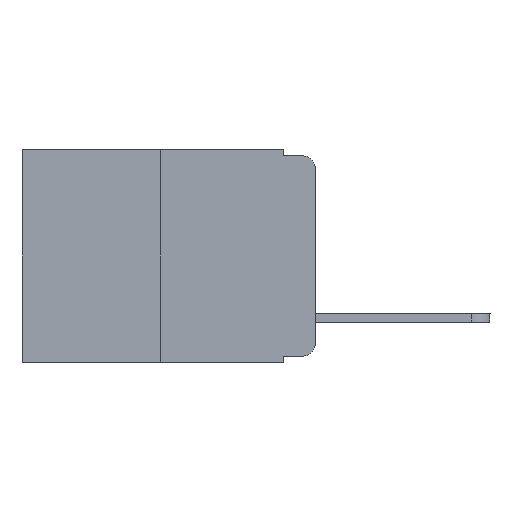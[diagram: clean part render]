
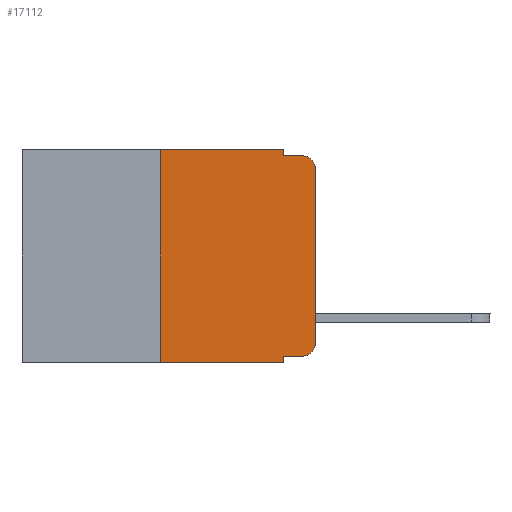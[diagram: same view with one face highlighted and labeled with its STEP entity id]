
A CAD part, left-side view. The second image highlights one B-rep face of the part: STEP entity #17112.
In plain terms, the highlighted planar face has unit normal (-1, 0, 0).
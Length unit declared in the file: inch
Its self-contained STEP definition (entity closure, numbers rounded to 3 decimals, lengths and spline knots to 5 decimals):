
#529 = CARTESIAN_POINT ( 'NONE',  ( 0., 0.051, -0.01 ) ) ;
#1294 = ORIENTED_EDGE ( 'NONE', *, *, #14803, .T. ) ;
#1505 = CIRCLE ( 'NONE', #15789, 0.02 ) ;
#2077 = CIRCLE ( 'NONE', #4795, 0.02 ) ;
#2731 = DIRECTION ( 'NONE',  ( 0., -1., 0. ) ) ;
#3553 = ORIENTED_EDGE ( 'NONE', *, *, #17590, .T. ) ;
#3739 = EDGE_LOOP ( 'NONE', ( #15089, #13191, #12401, #16859, #12333, #10802, #3553, #10987, #18357, #1294 ) ) ;
#4099 = DIRECTION ( 'NONE',  ( 0., 0., -1. ) ) ;
#4581 = VERTEX_POINT ( 'NONE', #529 ) ;
#4795 = AXIS2_PLACEMENT_3D ( 'NONE', #14480, #7601, #9352 ) ;
#4828 = DIRECTION ( 'NONE',  ( 0., 0., -1. ) ) ;
#4833 = CARTESIAN_POINT ( 'NONE',  ( 0., 0., -0.03 ) ) ;
#4875 = DIRECTION ( 'NONE',  ( 0., 0., -1. ) ) ;
#5605 = VECTOR ( 'NONE', #14605, 39.37008 ) ;
#5827 = CARTESIAN_POINT ( 'NONE',  ( 0., 0.25, 0. ) ) ;
#6003 = EDGE_CURVE ( 'NONE', #11993, #21894, #17107, .T. ) ;
#6407 = VERTEX_POINT ( 'NONE', #6464 ) ;
#6464 = CARTESIAN_POINT ( 'NONE',  ( 0., 0.02, -0.333 ) ) ;
#7314 = CARTESIAN_POINT ( 'NONE',  ( 0., 0.02, -0.313 ) ) ;
#7601 = DIRECTION ( 'NONE',  ( -1., 0., 0. ) ) ;
#7742 = VECTOR ( 'NONE', #12915, 39.37008 ) ;
#8338 = PLANE ( 'NONE',  #21215 ) ;
#9352 = DIRECTION ( 'NONE',  ( 0., 0., -1. ) ) ;
#9434 = DIRECTION ( 'NONE',  ( 0., -1., 0. ) ) ;
#9860 = EDGE_CURVE ( 'NONE', #4581, #17073, #19650, .T. ) ;
#9928 = VECTOR ( 'NONE', #18973, 39.37008 ) ;
#10130 = VERTEX_POINT ( 'NONE', #19594 ) ;
#10802 = ORIENTED_EDGE ( 'NONE', *, *, #18186, .F. ) ;
#10987 = ORIENTED_EDGE ( 'NONE', *, *, #6003, .F. ) ;
#11107 = CARTESIAN_POINT ( 'NONE',  ( 0., 0.473, -0.343 ) ) ;
#11209 = CARTESIAN_POINT ( 'NONE',  ( 0., 0.051, -0.333 ) ) ;
#11373 = VERTEX_POINT ( 'NONE', #4833 ) ;
#11555 = LINE ( 'NONE', #15477, #9928 ) ;
#11988 = VECTOR ( 'NONE', #4828, 39.37008 ) ;
#11993 = VERTEX_POINT ( 'NONE', #11209 ) ;
#12045 = CARTESIAN_POINT ( 'NONE',  ( 0., 0., -0.313 ) ) ;
#12333 = ORIENTED_EDGE ( 'NONE', *, *, #15250, .F. ) ;
#12401 = ORIENTED_EDGE ( 'NONE', *, *, #9860, .F. ) ;
#12915 = DIRECTION ( 'NONE',  ( 0., 0., 1. ) ) ;
#12977 = FACE_OUTER_BOUND ( 'NONE', #3739, .T. ) ;
#13163 = LINE ( 'NONE', #13746, #13716 ) ;
#13191 = ORIENTED_EDGE ( 'NONE', *, *, #17573, .T. ) ;
#13472 = CARTESIAN_POINT ( 'NONE',  ( 0., 0.473, 0. ) ) ;
#13675 = DIRECTION ( 'NONE',  ( 0., 0., -1. ) ) ;
#13716 = VECTOR ( 'NONE', #13675, 39.37008 ) ;
#13746 = CARTESIAN_POINT ( 'NONE',  ( 0., 0.051, 0. ) ) ;
#14480 = CARTESIAN_POINT ( 'NONE',  ( 0., 0.02, -0.03 ) ) ;
#14586 = CARTESIAN_POINT ( 'NONE',  ( 0., 0.051, -0.333 ) ) ;
#14605 = DIRECTION ( 'NONE',  ( 0., 0., 1. ) ) ;
#14635 = VERTEX_POINT ( 'NONE', #12045 ) ;
#14786 = CARTESIAN_POINT ( 'NONE',  ( 0., 0.051, 0. ) ) ;
#14803 = EDGE_CURVE ( 'NONE', #6407, #14635, #1505, .T. ) ;
#14926 = EDGE_CURVE ( 'NONE', #14635, #11373, #19141, .T. ) ;
#15005 = CARTESIAN_POINT ( 'NONE',  ( 0., 0.25, -0.343 ) ) ;
#15089 = ORIENTED_EDGE ( 'NONE', *, *, #14926, .T. ) ;
#15250 = EDGE_CURVE ( 'NONE', #10130, #17702, #11555, .T. ) ;
#15280 = EDGE_CURVE ( 'NONE', #17702, #4581, #13163, .T. ) ;
#15477 = CARTESIAN_POINT ( 'NONE',  ( 0., 0.473, 0. ) ) ;
#15673 = VERTEX_POINT ( 'NONE', #15005 ) ;
#15716 = CARTESIAN_POINT ( 'NONE',  ( 0., 0.051, -0.01 ) ) ;
#15789 = AXIS2_PLACEMENT_3D ( 'NONE', #7314, #16079, #4099 ) ;
#16079 = DIRECTION ( 'NONE',  ( -1., 0., 0. ) ) ;
#16113 = VECTOR ( 'NONE', #21182, 39.37008 ) ;
#16307 = CARTESIAN_POINT ( 'NONE',  ( 0., 0., 0. ) ) ;
#16730 = CARTESIAN_POINT ( 'NONE',  ( 0., 0.051, 0. ) ) ;
#16859 = ORIENTED_EDGE ( 'NONE', *, *, #15280, .F. ) ;
#17055 = EDGE_CURVE ( 'NONE', #11993, #6407, #18686, .T. ) ;
#17073 = VERTEX_POINT ( 'NONE', #20537 ) ;
#17107 = LINE ( 'NONE', #16730, #11988 ) ;
#17112 = ADVANCED_FACE ( 'NONE', ( #12977 ), #8338, .F. ) ;
#17563 = CARTESIAN_POINT ( 'NONE',  ( 0., 0.051, -0.343 ) ) ;
#17573 = EDGE_CURVE ( 'NONE', #11373, #17073, #2077, .T. ) ;
#17590 = EDGE_CURVE ( 'NONE', #15673, #21894, #21386, .T. ) ;
#17702 = VERTEX_POINT ( 'NONE', #14786 ) ;
#17797 = LINE ( 'NONE', #5827, #5605 ) ;
#18186 = EDGE_CURVE ( 'NONE', #15673, #10130, #17797, .T. ) ;
#18357 = ORIENTED_EDGE ( 'NONE', *, *, #17055, .T. ) ;
#18686 = LINE ( 'NONE', #14586, #22203 ) ;
#18973 = DIRECTION ( 'NONE',  ( 0., -1., 0. ) ) ;
#19141 = LINE ( 'NONE', #16307, #7742 ) ;
#19594 = CARTESIAN_POINT ( 'NONE',  ( 0., 0.25, 0. ) ) ;
#19650 = LINE ( 'NONE', #15716, #16113 ) ;
#20537 = CARTESIAN_POINT ( 'NONE',  ( 0., 0.02, -0.01 ) ) ;
#20855 = VECTOR ( 'NONE', #9434, 39.37008 ) ;
#21182 = DIRECTION ( 'NONE',  ( 0., -1., 0. ) ) ;
#21215 = AXIS2_PLACEMENT_3D ( 'NONE', #13472, #21953, #4875 ) ;
#21386 = LINE ( 'NONE', #11107, #20855 ) ;
#21894 = VERTEX_POINT ( 'NONE', #17563 ) ;
#21953 = DIRECTION ( 'NONE',  ( 1., 0., 0. ) ) ;
#22203 = VECTOR ( 'NONE', #2731, 39.37008 ) ;
